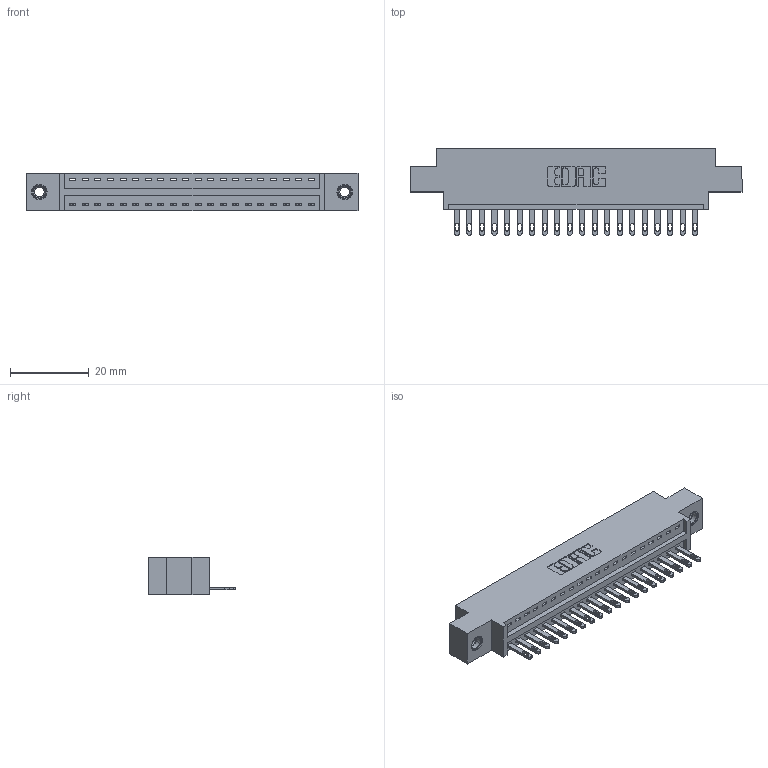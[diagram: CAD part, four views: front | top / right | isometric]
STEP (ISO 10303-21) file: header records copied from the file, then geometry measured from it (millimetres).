
FILE_DESCRIPTION (( 'STEP AP203' ), '1' );
FILE_NAME ('346-020-500-607.STEP', '2018-08-20T10:49:55', ( '' ), ( '' ), 'SwSTEP 2.0', 'SolidWorks 2016', '' );
FILE_SCHEMA (( 'CONFIG_CONTROL_DESIGN' ));
Length unit declared in the file: inch
Products named in the file (4): 346 Part_0.170 Offset - 0.156 Dia-TI; 345-292-001_345-293-100; 345-250-001_345-250-005-103; 346-020-500-607
Assembly tree (23 placements, depth 2):
  346-020-500-607
    346 Part_0.170 Offset - 0.156 Dia-TI
    345-292-001_345-293-100  x20
    345-250-001_345-250-005-103  x2
Bounding box: 84.07 x 21.84 x 9.4 mm (x, y, z)
Volume: 7740.4 mm3; surface area: 9678.7 mm2
Topology: 23 solids, 23 shells, 1266 faces, 3837 edges, 2550 vertices
Faces by surface type: plane 792, cylinder 458, cone 12, torus 4
Entity records: 16622 total; most frequent: CARTESIAN_POINT 2839, ORIENTED_EDGE 2786, DIRECTION 2559, EDGE_CURVE 1393, VECTOR 1157, LINE 1157, VERTEX_POINT 924, AXIS2_PLACEMENT_3D 701
